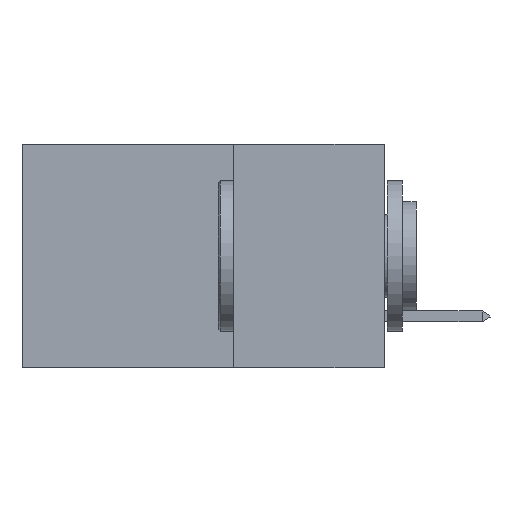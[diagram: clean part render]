
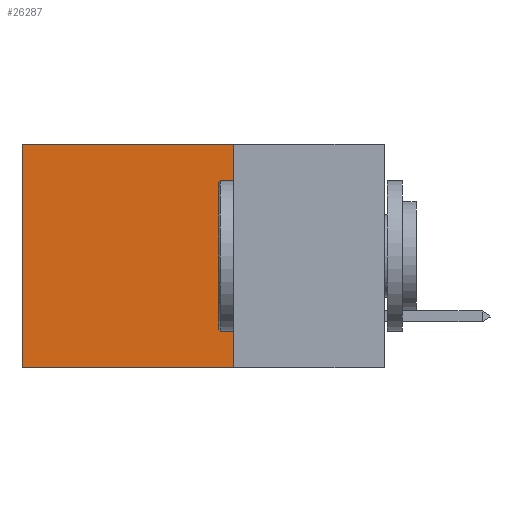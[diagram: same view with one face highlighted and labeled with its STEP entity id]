
A CAD part, left-side view. The second image highlights one B-rep face of the part: STEP entity #26287.
In plain terms, the highlighted planar face has unit normal (-1, 0, 0).
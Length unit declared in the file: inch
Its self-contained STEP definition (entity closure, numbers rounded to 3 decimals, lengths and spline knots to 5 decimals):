
#82 = DIRECTION ( 'NONE',  ( 0., 1., 0. ) ) ;
#1626 = DIRECTION ( 'NONE',  ( 0., 0., -1. ) ) ;
#2254 = CARTESIAN_POINT ( 'NONE',  ( 0.2875, 0.6, -0.37 ) ) ;
#2494 = CARTESIAN_POINT ( 'NONE',  ( 0.2875, 0.6, 0. ) ) ;
#2574 = CARTESIAN_POINT ( 'NONE',  ( 0.2875, 0.25, -0.37 ) ) ;
#2791 = DIRECTION ( 'NONE',  ( 0., 1., 0. ) ) ;
#3630 = FACE_OUTER_BOUND ( 'NONE', #5142, .T. ) ;
#4193 = VECTOR ( 'NONE', #82, 39.37008 ) ;
#4508 = CARTESIAN_POINT ( 'NONE',  ( 0.2875, 0.25, 0. ) ) ;
#4878 = VERTEX_POINT ( 'NONE', #29848 ) ;
#5142 = EDGE_LOOP ( 'NONE', ( #11322, #11911, #9976, #16546 ) ) ;
#5940 = DIRECTION ( 'NONE',  ( 1., 0., 0. ) ) ;
#6201 = LINE ( 'NONE', #4508, #20615 ) ;
#7786 = LINE ( 'NONE', #21220, #18482 ) ;
#8307 = PLANE ( 'NONE',  #24959 ) ;
#9134 = CARTESIAN_POINT ( 'NONE',  ( 0.2875, 0.25, -0.37 ) ) ;
#9716 = LINE ( 'NONE', #2574, #4193 ) ;
#9976 = ORIENTED_EDGE ( 'NONE', *, *, #19813, .F. ) ;
#11322 = ORIENTED_EDGE ( 'NONE', *, *, #18778, .T. ) ;
#11911 = ORIENTED_EDGE ( 'NONE', *, *, #14897, .F. ) ;
#12279 = VERTEX_POINT ( 'NONE', #13634 ) ;
#13634 = CARTESIAN_POINT ( 'NONE',  ( 0.2875, 0.25, 0. ) ) ;
#14897 = EDGE_CURVE ( 'NONE', #15977, #23693, #9716, .T. ) ;
#15712 = CARTESIAN_POINT ( 'NONE',  ( 0.2875, 0.25, 0. ) ) ;
#15977 = VERTEX_POINT ( 'NONE', #9134 ) ;
#16546 = ORIENTED_EDGE ( 'NONE', *, *, #28908, .T. ) ;
#16973 = DIRECTION ( 'NONE',  ( 0., 0., -1. ) ) ;
#18482 = VECTOR ( 'NONE', #2791, 39.37008 ) ;
#18778 = EDGE_CURVE ( 'NONE', #4878, #23693, #27557, .T. ) ;
#19813 = EDGE_CURVE ( 'NONE', #12279, #15977, #6201, .T. ) ;
#20615 = VECTOR ( 'NONE', #20683, 39.37008 ) ;
#20683 = DIRECTION ( 'NONE',  ( 0., 0., -1. ) ) ;
#21220 = CARTESIAN_POINT ( 'NONE',  ( 0.2875, 0.25, 0. ) ) ;
#23693 = VERTEX_POINT ( 'NONE', #2254 ) ;
#24959 = AXIS2_PLACEMENT_3D ( 'NONE', #15712, #5940, #1626 ) ;
#26287 = ADVANCED_FACE ( 'NONE', ( #3630 ), #8307, .F. ) ;
#27557 = LINE ( 'NONE', #2494, #29022 ) ;
#28908 = EDGE_CURVE ( 'NONE', #12279, #4878, #7786, .T. ) ;
#29022 = VECTOR ( 'NONE', #16973, 39.37008 ) ;
#29848 = CARTESIAN_POINT ( 'NONE',  ( 0.2875, 0.6, 0. ) ) ;
